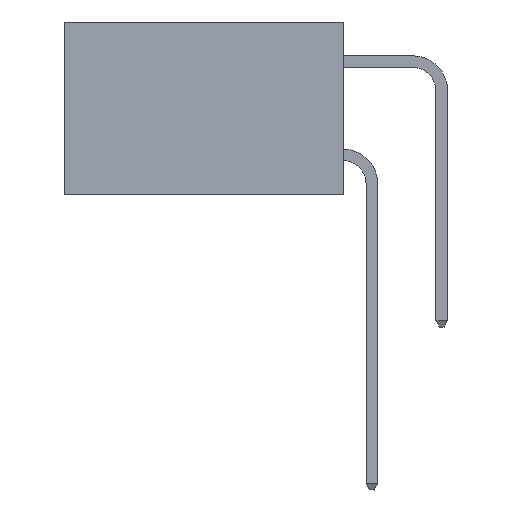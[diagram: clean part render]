
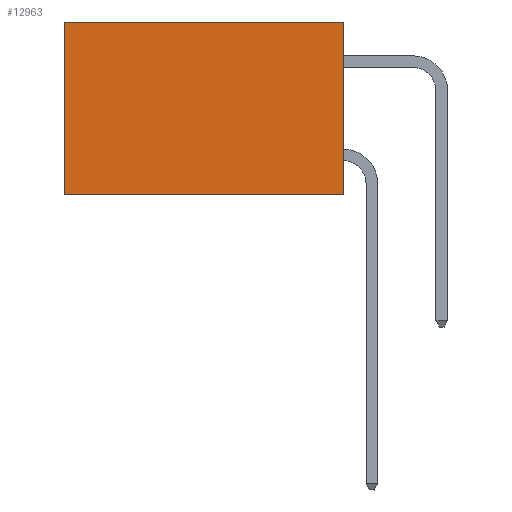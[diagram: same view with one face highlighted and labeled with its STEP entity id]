
A CAD part, left-side view. The second image highlights one B-rep face of the part: STEP entity #12963.
In plain terms, the highlighted planar face has unit normal (-1, 0, 0).
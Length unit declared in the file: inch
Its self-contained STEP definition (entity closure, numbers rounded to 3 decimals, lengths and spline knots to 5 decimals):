
#439 = FACE_OUTER_BOUND ( 'NONE', #7547, .T. ) ;
#1486 = DIRECTION ( 'NONE',  ( 0., 1., 0. ) ) ;
#2004 = DIRECTION ( 'NONE',  ( 0., 0., -1. ) ) ;
#2480 = VERTEX_POINT ( 'NONE', #9859 ) ;
#3398 = VECTOR ( 'NONE', #7838, 39.37008 ) ;
#3768 = PLANE ( 'NONE',  #22091 ) ;
#6376 = CARTESIAN_POINT ( 'NONE',  ( 0.298, 0.6, 0. ) ) ;
#6766 = LINE ( 'NONE', #17880, #15761 ) ;
#7547 = EDGE_LOOP ( 'NONE', ( #17999, #12634, #14846, #13336 ) ) ;
#7748 = VERTEX_POINT ( 'NONE', #22696 ) ;
#7838 = DIRECTION ( 'NONE',  ( 0., 1., 0. ) ) ;
#8080 = LINE ( 'NONE', #22822, #12296 ) ;
#9165 = CARTESIAN_POINT ( 'NONE',  ( 0.298, 0., 0. ) ) ;
#9859 = CARTESIAN_POINT ( 'NONE',  ( 0.298, 0.6, -0.37 ) ) ;
#12018 = CARTESIAN_POINT ( 'NONE',  ( 0.298, 0., 0. ) ) ;
#12296 = VECTOR ( 'NONE', #1486, 39.37008 ) ;
#12536 = VECTOR ( 'NONE', #18908, 39.37008 ) ;
#12634 = ORIENTED_EDGE ( 'NONE', *, *, #21533, .F. ) ;
#12782 = DIRECTION ( 'NONE',  ( 1., 0., 0. ) ) ;
#12963 = ADVANCED_FACE ( 'NONE', ( #439 ), #3768, .F. ) ;
#13336 = ORIENTED_EDGE ( 'NONE', *, *, #19789, .T. ) ;
#14685 = VERTEX_POINT ( 'NONE', #12018 ) ;
#14846 = ORIENTED_EDGE ( 'NONE', *, *, #19658, .F. ) ;
#15723 = CARTESIAN_POINT ( 'NONE',  ( 0.298, 0.6, 0. ) ) ;
#15761 = VECTOR ( 'NONE', #17959, 39.37008 ) ;
#16787 = CARTESIAN_POINT ( 'NONE',  ( 0.298, 0., 0. ) ) ;
#17326 = LINE ( 'NONE', #6376, #12536 ) ;
#17709 = LINE ( 'NONE', #16787, #3398 ) ;
#17880 = CARTESIAN_POINT ( 'NONE',  ( 0.298, 0., 0. ) ) ;
#17957 = VERTEX_POINT ( 'NONE', #15723 ) ;
#17959 = DIRECTION ( 'NONE',  ( 0., 0., -1. ) ) ;
#17999 = ORIENTED_EDGE ( 'NONE', *, *, #21981, .T. ) ;
#18908 = DIRECTION ( 'NONE',  ( 0., 0., -1. ) ) ;
#19658 = EDGE_CURVE ( 'NONE', #14685, #7748, #6766, .T. ) ;
#19789 = EDGE_CURVE ( 'NONE', #14685, #17957, #17709, .T. ) ;
#21533 = EDGE_CURVE ( 'NONE', #7748, #2480, #8080, .T. ) ;
#21981 = EDGE_CURVE ( 'NONE', #17957, #2480, #17326, .T. ) ;
#22091 = AXIS2_PLACEMENT_3D ( 'NONE', #9165, #12782, #2004 ) ;
#22696 = CARTESIAN_POINT ( 'NONE',  ( 0.298, 0., -0.37 ) ) ;
#22822 = CARTESIAN_POINT ( 'NONE',  ( 0.298, 0., -0.37 ) ) ;
